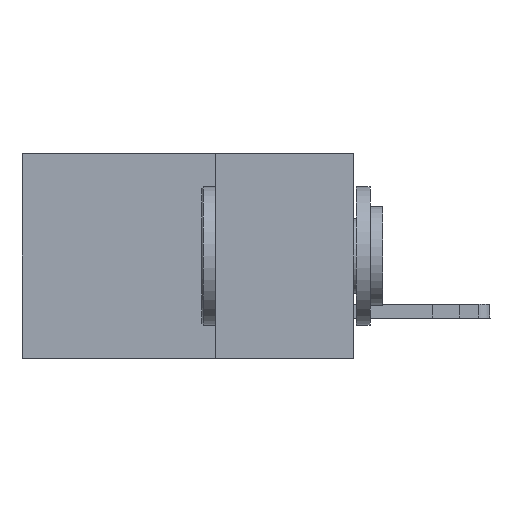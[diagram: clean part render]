
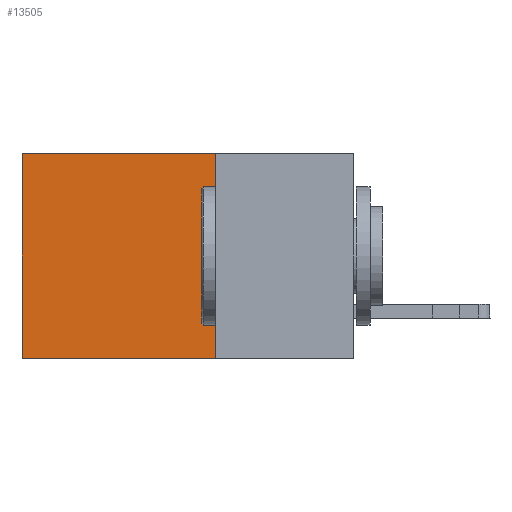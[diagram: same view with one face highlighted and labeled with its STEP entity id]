
A CAD part, left-side view. The second image highlights one B-rep face of the part: STEP entity #13505.
In plain terms, the highlighted planar face has unit normal (-1, 0, 0).
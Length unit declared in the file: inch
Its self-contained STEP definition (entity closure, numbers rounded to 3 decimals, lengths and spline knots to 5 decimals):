
#69 = FACE_OUTER_BOUND ( 'NONE', #16421, .T. ) ;
#753 = ORIENTED_EDGE ( 'NONE', *, *, #1717, .T. ) ;
#1640 = DIRECTION ( 'NONE',  ( 0., 0., -1. ) ) ;
#1717 = EDGE_CURVE ( 'NONE', #7768, #7251, #11984, .T. ) ;
#1932 = CARTESIAN_POINT ( 'NONE',  ( 0.2875, 0.25, 0. ) ) ;
#2557 = VECTOR ( 'NONE', #9986, 39.37008 ) ;
#2946 = DIRECTION ( 'NONE',  ( 0., 1., 0. ) ) ;
#4249 = LINE ( 'NONE', #8112, #17001 ) ;
#4800 = CARTESIAN_POINT ( 'NONE',  ( 0.2875, 0.25, -0.37 ) ) ;
#5292 = CARTESIAN_POINT ( 'NONE',  ( 0.2875, 0.6, 0. ) ) ;
#5295 = EDGE_CURVE ( 'NONE', #14169, #14040, #16397, .T. ) ;
#6502 = CARTESIAN_POINT ( 'NONE',  ( 0.2875, 0.25, 0. ) ) ;
#6579 = VECTOR ( 'NONE', #15792, 39.37008 ) ;
#7008 = AXIS2_PLACEMENT_3D ( 'NONE', #20573, #12036, #1640 ) ;
#7251 = VERTEX_POINT ( 'NONE', #17270 ) ;
#7368 = VECTOR ( 'NONE', #20465, 39.37008 ) ;
#7768 = VERTEX_POINT ( 'NONE', #5292 ) ;
#8025 = ORIENTED_EDGE ( 'NONE', *, *, #5295, .F. ) ;
#8112 = CARTESIAN_POINT ( 'NONE',  ( 0.2875, 0.25, -0.37 ) ) ;
#9986 = DIRECTION ( 'NONE',  ( 0., 0., -1. ) ) ;
#10344 = CARTESIAN_POINT ( 'NONE',  ( 0.2875, 0.25, 0. ) ) ;
#11717 = LINE ( 'NONE', #1932, #6579 ) ;
#11984 = LINE ( 'NONE', #20653, #7368 ) ;
#12036 = DIRECTION ( 'NONE',  ( 1., 0., 0. ) ) ;
#13505 = ADVANCED_FACE ( 'NONE', ( #69 ), #13688, .F. ) ;
#13620 = EDGE_CURVE ( 'NONE', #14169, #7768, #11717, .T. ) ;
#13688 = PLANE ( 'NONE',  #7008 ) ;
#14040 = VERTEX_POINT ( 'NONE', #4800 ) ;
#14169 = VERTEX_POINT ( 'NONE', #10344 ) ;
#15792 = DIRECTION ( 'NONE',  ( 0., 1., 0. ) ) ;
#16397 = LINE ( 'NONE', #6502, #2557 ) ;
#16421 = EDGE_LOOP ( 'NONE', ( #753, #21159, #8025, #21636 ) ) ;
#17001 = VECTOR ( 'NONE', #2946, 39.37008 ) ;
#17270 = CARTESIAN_POINT ( 'NONE',  ( 0.2875, 0.6, -0.37 ) ) ;
#20188 = EDGE_CURVE ( 'NONE', #14040, #7251, #4249, .T. ) ;
#20465 = DIRECTION ( 'NONE',  ( 0., 0., -1. ) ) ;
#20573 = CARTESIAN_POINT ( 'NONE',  ( 0.2875, 0.25, 0. ) ) ;
#20653 = CARTESIAN_POINT ( 'NONE',  ( 0.2875, 0.6, 0. ) ) ;
#21159 = ORIENTED_EDGE ( 'NONE', *, *, #20188, .F. ) ;
#21636 = ORIENTED_EDGE ( 'NONE', *, *, #13620, .T. ) ;
